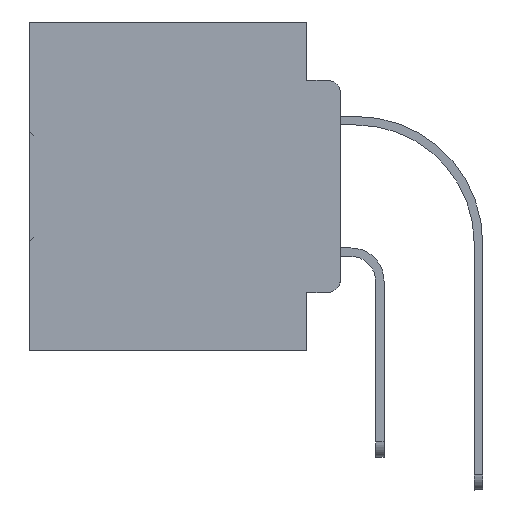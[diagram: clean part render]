
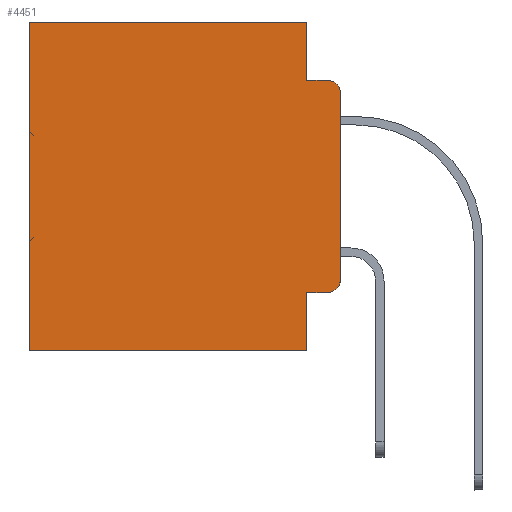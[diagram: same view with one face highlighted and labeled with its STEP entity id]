
A CAD part, left-side view. The second image highlights one B-rep face of the part: STEP entity #4451.
In plain terms, the highlighted planar face has unit normal (-1, 0, 0).
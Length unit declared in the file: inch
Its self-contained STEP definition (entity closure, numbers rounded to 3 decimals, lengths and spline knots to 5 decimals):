
#991 = LINE ( 'NONE', #3677, #4435 ) ;
#1049 = VERTEX_POINT ( 'NONE', #26404 ) ;
#1204 = CIRCLE ( 'NONE', #32348, 0.02 ) ;
#2618 = FACE_OUTER_BOUND ( 'NONE', #10882, .T. ) ;
#2645 = CARTESIAN_POINT ( 'NONE',  ( 0.298, 0.02, -0.1085 ) ) ;
#3549 = ORIENTED_EDGE ( 'NONE', *, *, #12370, .T. ) ;
#3677 = CARTESIAN_POINT ( 'NONE',  ( 0.298, 0., -0.5 ) ) ;
#3734 = CARTESIAN_POINT ( 'NONE',  ( 0.298, 0., -0.1085 ) ) ;
#3777 = CARTESIAN_POINT ( 'NONE',  ( 0.298, 0.051, 0. ) ) ;
#3801 = LINE ( 'NONE', #15262, #32833 ) ;
#3918 = EDGE_CURVE ( 'NONE', #30748, #1049, #5393, .T. ) ;
#4435 = VECTOR ( 'NONE', #24139, 39.37008 ) ;
#4451 = ADVANCED_FACE ( 'NONE', ( #2618 ), #25953, .F. ) ;
#4927 = ORIENTED_EDGE ( 'NONE', *, *, #27524, .T. ) ;
#5308 = DIRECTION ( 'NONE',  ( 0., 0., -1. ) ) ;
#5331 = VECTOR ( 'NONE', #13994, 39.37008 ) ;
#5393 = LINE ( 'NONE', #23162, #5331 ) ;
#5562 = DIRECTION ( 'NONE',  ( 0., 0., -1. ) ) ;
#5626 = CARTESIAN_POINT ( 'NONE',  ( 0.298, 0., -0.3915 ) ) ;
#6075 = ORIENTED_EDGE ( 'NONE', *, *, #29005, .T. ) ;
#7520 = DIRECTION ( 'NONE',  ( 0., 0., -1. ) ) ;
#9073 = EDGE_CURVE ( 'NONE', #37654, #34131, #28719, .T. ) ;
#9865 = ORIENTED_EDGE ( 'NONE', *, *, #14555, .T. ) ;
#10793 = LINE ( 'NONE', #16576, #36563 ) ;
#10882 = EDGE_LOOP ( 'NONE', ( #35246, #9865, #13841, #24399, #6075, #4927, #28598, #13366, #3549, #21702 ) ) ;
#11210 = CARTESIAN_POINT ( 'NONE',  ( 0.298, 0., 0. ) ) ;
#11377 = DIRECTION ( 'NONE',  ( 1., 0., 0. ) ) ;
#12068 = AXIS2_PLACEMENT_3D ( 'NONE', #11210, #11377, #34383 ) ;
#12370 = EDGE_CURVE ( 'NONE', #30748, #24191, #3801, .T. ) ;
#12566 = DIRECTION ( 'NONE',  ( 0., -1., 0. ) ) ;
#13366 = ORIENTED_EDGE ( 'NONE', *, *, #3918, .F. ) ;
#13692 = DIRECTION ( 'NONE',  ( 0., -1., 0. ) ) ;
#13841 = ORIENTED_EDGE ( 'NONE', *, *, #36073, .F. ) ;
#13994 = DIRECTION ( 'NONE',  ( 0., 0., -1. ) ) ;
#14555 = EDGE_CURVE ( 'NONE', #15208, #19452, #34409, .T. ) ;
#15208 = VERTEX_POINT ( 'NONE', #3734 ) ;
#15262 = CARTESIAN_POINT ( 'NONE',  ( 0.298, 0.051, -0.4115 ) ) ;
#16576 = CARTESIAN_POINT ( 'NONE',  ( 0.298, 0.051, -0.0885 ) ) ;
#16684 = CARTESIAN_POINT ( 'NONE',  ( 0.298, 0., 0. ) ) ;
#16715 = CARTESIAN_POINT ( 'NONE',  ( 0.298, 0.473, 0. ) ) ;
#19452 = VERTEX_POINT ( 'NONE', #36799 ) ;
#19521 = VERTEX_POINT ( 'NONE', #20501 ) ;
#19742 = EDGE_CURVE ( 'NONE', #1049, #35643, #991, .T. ) ;
#19774 = EDGE_CURVE ( 'NONE', #15208, #22672, #36758, .T. ) ;
#20225 = CARTESIAN_POINT ( 'NONE',  ( 0.298, 0.02, -0.4115 ) ) ;
#20228 = DIRECTION ( 'NONE',  ( -1., 0., 0. ) ) ;
#20309 = VECTOR ( 'NONE', #5562, 39.37008 ) ;
#20501 = CARTESIAN_POINT ( 'NONE',  ( 0.298, 0.473, 0. ) ) ;
#21702 = ORIENTED_EDGE ( 'NONE', *, *, #29768, .T. ) ;
#22672 = VERTEX_POINT ( 'NONE', #5626 ) ;
#22897 = DIRECTION ( 'NONE',  ( -1., 0., 0. ) ) ;
#23130 = VECTOR ( 'NONE', #31997, 39.37008 ) ;
#23162 = CARTESIAN_POINT ( 'NONE',  ( 0.298, 0.051, 0. ) ) ;
#24139 = DIRECTION ( 'NONE',  ( 0., 1., 0. ) ) ;
#24191 = VERTEX_POINT ( 'NONE', #20225 ) ;
#24399 = ORIENTED_EDGE ( 'NONE', *, *, #9073, .F. ) ;
#25953 = PLANE ( 'NONE',  #12068 ) ;
#26404 = CARTESIAN_POINT ( 'NONE',  ( 0.298, 0.051, -0.5 ) ) ;
#26598 = CARTESIAN_POINT ( 'NONE',  ( 0.298, 0.051, -0.4115 ) ) ;
#27524 = EDGE_CURVE ( 'NONE', #19521, #35643, #36959, .T. ) ;
#27743 = CARTESIAN_POINT ( 'NONE',  ( 0.298, 0.051, -0.0885 ) ) ;
#28354 = CARTESIAN_POINT ( 'NONE',  ( 0.298, 0.473, -0.5 ) ) ;
#28598 = ORIENTED_EDGE ( 'NONE', *, *, #19742, .F. ) ;
#28719 = LINE ( 'NONE', #37499, #20309 ) ;
#28931 = AXIS2_PLACEMENT_3D ( 'NONE', #2645, #22897, #33703 ) ;
#29005 = EDGE_CURVE ( 'NONE', #37654, #19521, #31804, .T. ) ;
#29768 = EDGE_CURVE ( 'NONE', #24191, #22672, #1204, .T. ) ;
#30748 = VERTEX_POINT ( 'NONE', #26598 ) ;
#31804 = LINE ( 'NONE', #34857, #23130 ) ;
#31997 = DIRECTION ( 'NONE',  ( 0., 1., 0. ) ) ;
#32348 = AXIS2_PLACEMENT_3D ( 'NONE', #34565, #20228, #5308 ) ;
#32833 = VECTOR ( 'NONE', #12566, 39.37008 ) ;
#33703 = DIRECTION ( 'NONE',  ( 0., 0., -1. ) ) ;
#33752 = VECTOR ( 'NONE', #7520, 39.37008 ) ;
#34131 = VERTEX_POINT ( 'NONE', #27743 ) ;
#34383 = DIRECTION ( 'NONE',  ( 0., 0., -1. ) ) ;
#34409 = CIRCLE ( 'NONE', #28931, 0.02 ) ;
#34565 = CARTESIAN_POINT ( 'NONE',  ( 0.298, 0.02, -0.3915 ) ) ;
#34857 = CARTESIAN_POINT ( 'NONE',  ( 0.298, 0., 0. ) ) ;
#35246 = ORIENTED_EDGE ( 'NONE', *, *, #19774, .F. ) ;
#35643 = VERTEX_POINT ( 'NONE', #28354 ) ;
#36040 = VECTOR ( 'NONE', #37143, 39.37008 ) ;
#36073 = EDGE_CURVE ( 'NONE', #34131, #19452, #10793, .T. ) ;
#36563 = VECTOR ( 'NONE', #13692, 39.37008 ) ;
#36758 = LINE ( 'NONE', #16684, #33752 ) ;
#36799 = CARTESIAN_POINT ( 'NONE',  ( 0.298, 0.02, -0.0885 ) ) ;
#36959 = LINE ( 'NONE', #16715, #36040 ) ;
#37143 = DIRECTION ( 'NONE',  ( 0., 0., -1. ) ) ;
#37499 = CARTESIAN_POINT ( 'NONE',  ( 0.298, 0.051, 0. ) ) ;
#37654 = VERTEX_POINT ( 'NONE', #3777 ) ;
